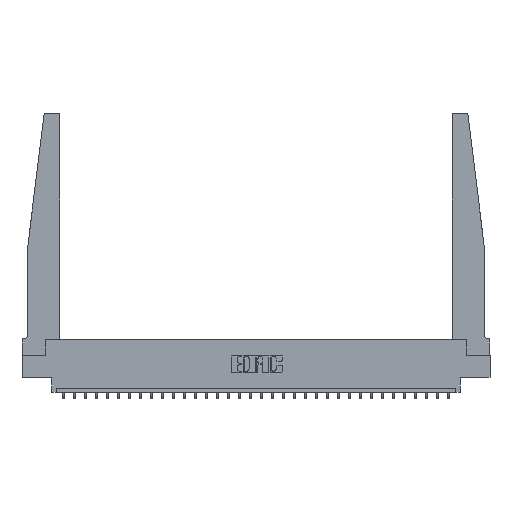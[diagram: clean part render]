
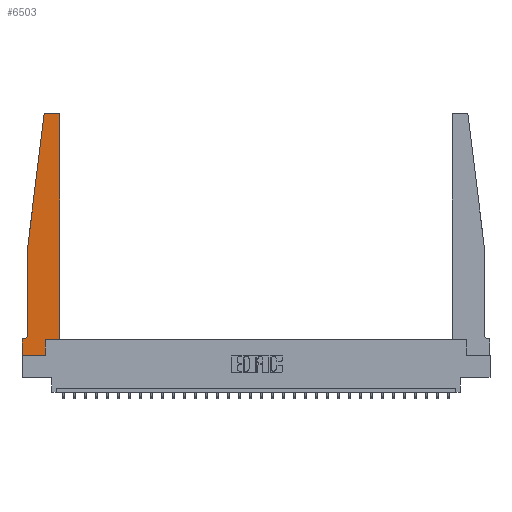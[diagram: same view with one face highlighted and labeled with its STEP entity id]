
A CAD part, top view. The second image highlights one B-rep face of the part: STEP entity #6503.
In plain terms, the highlighted planar face has unit normal (0, 0, 1).
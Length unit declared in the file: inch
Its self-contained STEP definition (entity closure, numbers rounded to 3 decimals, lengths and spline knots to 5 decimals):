
#117 = EDGE_CURVE ( 'NONE', #6763, #501, #10268, .T. ) ;
#501 = VERTEX_POINT ( 'NONE', #1389 ) ;
#519 = CARTESIAN_POINT ( 'NONE',  ( 0., 0., 0.37 ) ) ;
#559 = EDGE_CURVE ( 'NONE', #17113, #9757, #28134, .T. ) ;
#634 = DIRECTION ( 'NONE',  ( 1., 0., 0. ) ) ;
#699 = DIRECTION ( 'NONE',  ( -1., 0., 0. ) ) ;
#908 = DIRECTION ( 'NONE',  ( -1., 0., 0. ) ) ;
#1091 = CARTESIAN_POINT ( 'NONE',  ( 0.2605, 0.18, 0.37 ) ) ;
#1389 = CARTESIAN_POINT ( 'NONE',  ( 0.2605, 0., 0.37 ) ) ;
#1532 = EDGE_CURVE ( 'NONE', #19833, #20693, #26733, .T. ) ;
#2021 = CARTESIAN_POINT ( 'NONE',  ( 0.24675, 2.72367, 0.37 ) ) ;
#2180 = DIRECTION ( 'NONE',  ( 1., 0., 0. ) ) ;
#2233 = DIRECTION ( 'NONE',  ( 0., 0., 1. ) ) ;
#2238 = VERTEX_POINT ( 'NONE', #24247 ) ;
#2743 = DIRECTION ( 'NONE',  ( 0., -1., 0. ) ) ;
#3174 = CARTESIAN_POINT ( 'NONE',  ( 0., 0., 0.37 ) ) ;
#3407 = VECTOR ( 'NONE', #2743, 39.37008 ) ;
#3731 = ORIENTED_EDGE ( 'NONE', *, *, #25911, .T. ) ;
#3994 = DIRECTION ( 'NONE',  ( 0., 0., 1. ) ) ;
#4082 = LINE ( 'NONE', #519, #3407 ) ;
#4143 = CARTESIAN_POINT ( 'NONE',  ( 0.065, 1.25, 0.37 ) ) ;
#4223 = DIRECTION ( 'NONE',  ( 0., -1., 0. ) ) ;
#4428 = VECTOR ( 'NONE', #2180, 39.37008 ) ;
#5216 = ORIENTED_EDGE ( 'NONE', *, *, #8175, .T. ) ;
#5642 = ORIENTED_EDGE ( 'NONE', *, *, #26817, .T. ) ;
#5800 = LINE ( 'NONE', #15062, #16657 ) ;
#6107 = CARTESIAN_POINT ( 'NONE',  ( 0., 0.1875, 0.37 ) ) ;
#6186 = VECTOR ( 'NONE', #14159, 39.37008 ) ;
#6503 = ADVANCED_FACE ( 'NONE', ( #26474 ), #16823, .T. ) ;
#6763 = VERTEX_POINT ( 'NONE', #9138 ) ;
#6774 = VERTEX_POINT ( 'NONE', #26441 ) ;
#6819 = VECTOR ( 'NONE', #10025, 39.37008 ) ;
#6843 = ORIENTED_EDGE ( 'NONE', *, *, #24118, .T. ) ;
#7381 = EDGE_CURVE ( 'NONE', #10959, #6774, #5800, .T. ) ;
#7462 = DIRECTION ( 'NONE',  ( -1., 0., 0. ) ) ;
#8020 = LINE ( 'NONE', #10337, #18855 ) ;
#8175 = EDGE_CURVE ( 'NONE', #6774, #17113, #19984, .T. ) ;
#8395 = VERTEX_POINT ( 'NONE', #25608 ) ;
#9138 = CARTESIAN_POINT ( 'NONE',  ( 0., 0., 0.37 ) ) ;
#9328 = CARTESIAN_POINT ( 'NONE',  ( 0.425, 2.72, 0.37 ) ) ;
#9757 = VERTEX_POINT ( 'NONE', #10781 ) ;
#10025 = DIRECTION ( 'NONE',  ( -0.122, -0.992, 0. ) ) ;
#10069 = EDGE_LOOP ( 'NONE', ( #6843, #22334, #19665, #25283, #5216, #14886, #3731, #18466, #21527, #19437, #5642, #25537 ) ) ;
#10191 = EDGE_CURVE ( 'NONE', #20693, #10959, #16996, .T. ) ;
#10268 = LINE ( 'NONE', #3174, #4428 ) ;
#10337 = CARTESIAN_POINT ( 'NONE',  ( 0.425, 0.18, 0.37 ) ) ;
#10506 = CARTESIAN_POINT ( 'NONE',  ( 0.015, 0.1875, 0.37 ) ) ;
#10781 = CARTESIAN_POINT ( 'NONE',  ( 0., 0.1875, 0.37 ) ) ;
#10902 = VECTOR ( 'NONE', #7462, 39.37008 ) ;
#10959 = VERTEX_POINT ( 'NONE', #4143 ) ;
#11202 = LINE ( 'NONE', #22652, #22029 ) ;
#11414 = AXIS2_PLACEMENT_3D ( 'NONE', #26936, #13983, #908 ) ;
#13685 = DIRECTION ( 'NONE',  ( 0., 0., 1. ) ) ;
#13983 = DIRECTION ( 'NONE',  ( 0., 0., -1. ) ) ;
#14159 = DIRECTION ( 'NONE',  ( 0., 1., 0. ) ) ;
#14886 = ORIENTED_EDGE ( 'NONE', *, *, #559, .T. ) ;
#15062 = CARTESIAN_POINT ( 'NONE',  ( 0.065, 1.25, 0.37 ) ) ;
#15067 = LINE ( 'NONE', #26720, #25894 ) ;
#15272 = CARTESIAN_POINT ( 'NONE',  ( 0.27653, 2.72, 0.37 ) ) ;
#15771 = VERTEX_POINT ( 'NONE', #23068 ) ;
#16508 = AXIS2_PLACEMENT_3D ( 'NONE', #6107, #3994, #19181 ) ;
#16657 = VECTOR ( 'NONE', #4223, 39.37008 ) ;
#16739 = AXIS2_PLACEMENT_3D ( 'NONE', #26663, #13685, #634 ) ;
#16823 = PLANE ( 'NONE',  #16508 ) ;
#16996 = LINE ( 'NONE', #22987, #6819 ) ;
#17048 = EDGE_CURVE ( 'NONE', #8395, #15771, #8020, .T. ) ;
#17113 = VERTEX_POINT ( 'NONE', #10506 ) ;
#17434 = DIRECTION ( 'NONE',  ( 1., 0., 0. ) ) ;
#18466 = ORIENTED_EDGE ( 'NONE', *, *, #117, .T. ) ;
#18539 = VERTEX_POINT ( 'NONE', #9328 ) ;
#18804 = AXIS2_PLACEMENT_3D ( 'NONE', #15272, #2233, #17434 ) ;
#18855 = VECTOR ( 'NONE', #27420, 39.37008 ) ;
#19181 = DIRECTION ( 'NONE',  ( 1., 0., 0. ) ) ;
#19437 = ORIENTED_EDGE ( 'NONE', *, *, #17048, .T. ) ;
#19665 = ORIENTED_EDGE ( 'NONE', *, *, #10191, .T. ) ;
#19833 = VERTEX_POINT ( 'NONE', #24678 ) ;
#19935 = EDGE_CURVE ( 'NONE', #501, #8395, #23487, .T. ) ;
#19984 = CIRCLE ( 'NONE', #11414, 0.05 ) ;
#20693 = VERTEX_POINT ( 'NONE', #2021 ) ;
#21527 = ORIENTED_EDGE ( 'NONE', *, *, #19935, .T. ) ;
#22029 = VECTOR ( 'NONE', #24822, 39.37008 ) ;
#22334 = ORIENTED_EDGE ( 'NONE', *, *, #1532, .T. ) ;
#22652 = CARTESIAN_POINT ( 'NONE',  ( 0.425, 0.18, 0.37 ) ) ;
#22975 = CARTESIAN_POINT ( 'NONE',  ( 0.065, 0.1875, 0.37 ) ) ;
#22987 = CARTESIAN_POINT ( 'NONE',  ( 0.065, 1.25, 0.37 ) ) ;
#23068 = CARTESIAN_POINT ( 'NONE',  ( 0.425, 0.18, 0.37 ) ) ;
#23487 = LINE ( 'NONE', #1091, #6186 ) ;
#24118 = EDGE_CURVE ( 'NONE', #2238, #19833, #15067, .T. ) ;
#24247 = CARTESIAN_POINT ( 'NONE',  ( 0.395, 2.75, 0.37 ) ) ;
#24678 = CARTESIAN_POINT ( 'NONE',  ( 0.27653, 2.75, 0.37 ) ) ;
#24822 = DIRECTION ( 'NONE',  ( 0., 1., 0. ) ) ;
#25283 = ORIENTED_EDGE ( 'NONE', *, *, #7381, .T. ) ;
#25418 = EDGE_CURVE ( 'NONE', #18539, #2238, #27173, .T. ) ;
#25537 = ORIENTED_EDGE ( 'NONE', *, *, #25418, .T. ) ;
#25608 = CARTESIAN_POINT ( 'NONE',  ( 0.2605, 0.18, 0.37 ) ) ;
#25894 = VECTOR ( 'NONE', #699, 39.37008 ) ;
#25911 = EDGE_CURVE ( 'NONE', #9757, #6763, #4082, .T. ) ;
#26441 = CARTESIAN_POINT ( 'NONE',  ( 0.065, 0.2375, 0.37 ) ) ;
#26474 = FACE_OUTER_BOUND ( 'NONE', #10069, .T. ) ;
#26663 = CARTESIAN_POINT ( 'NONE',  ( 0.395, 2.72, 0.37 ) ) ;
#26720 = CARTESIAN_POINT ( 'NONE',  ( 0.25, 2.75, 0.37 ) ) ;
#26733 = CIRCLE ( 'NONE', #18804, 0.03 ) ;
#26817 = EDGE_CURVE ( 'NONE', #15771, #18539, #11202, .T. ) ;
#26936 = CARTESIAN_POINT ( 'NONE',  ( 0.015, 0.2375, 0.37 ) ) ;
#27173 = CIRCLE ( 'NONE', #16739, 0.03 ) ;
#27420 = DIRECTION ( 'NONE',  ( 1., 0., 0. ) ) ;
#28134 = LINE ( 'NONE', #22975, #10902 ) ;
